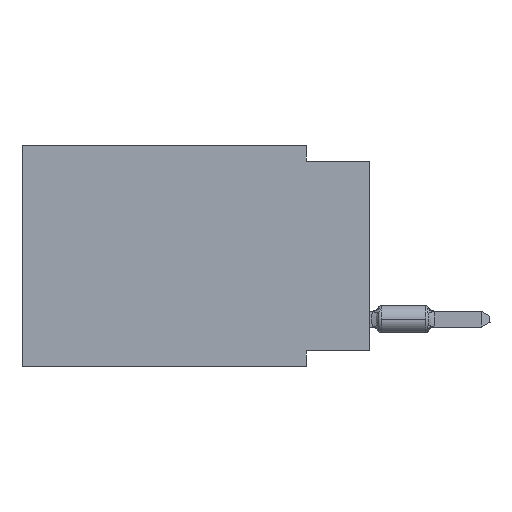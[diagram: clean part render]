
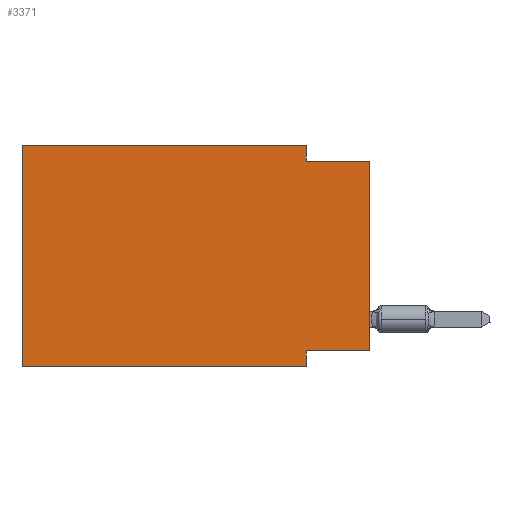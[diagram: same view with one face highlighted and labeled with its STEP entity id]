
A CAD part, left-side view. The second image highlights one B-rep face of the part: STEP entity #3371.
In plain terms, the highlighted planar face has unit normal (-1, 0, 0).
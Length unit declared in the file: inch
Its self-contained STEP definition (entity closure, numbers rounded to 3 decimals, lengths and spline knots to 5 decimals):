
#1636 = LINE ( 'NONE', #6308, #57875 ) ;
#3371 = ADVANCED_FACE ( 'NONE', ( #10774 ), #32274, .F. ) ;
#4884 = CARTESIAN_POINT ( 'NONE',  ( 0., 0., -0.325 ) ) ;
#5428 = DIRECTION ( 'NONE',  ( 0., 0., -1. ) ) ;
#6308 = CARTESIAN_POINT ( 'NONE',  ( 0., 0.55, -0.35 ) ) ;
#6967 = ORIENTED_EDGE ( 'NONE', *, *, #47789, .T. ) ;
#7202 = CARTESIAN_POINT ( 'NONE',  ( 0., 0.1, -0.35 ) ) ;
#7401 = CARTESIAN_POINT ( 'NONE',  ( 0., 0., -0.025 ) ) ;
#8218 = VECTOR ( 'NONE', #26713, 39.37008 ) ;
#8682 = DIRECTION ( 'NONE',  ( 0., -1., 0. ) ) ;
#9375 = DIRECTION ( 'NONE',  ( 0., 0., 1. ) ) ;
#9652 = VERTEX_POINT ( 'NONE', #34752 ) ;
#9842 = EDGE_CURVE ( 'NONE', #9652, #63638, #1636, .T. ) ;
#10419 = CARTESIAN_POINT ( 'NONE',  ( 0., 0., 0. ) ) ;
#10774 = FACE_OUTER_BOUND ( 'NONE', #28604, .T. ) ;
#10918 = EDGE_CURVE ( 'NONE', #28809, #63638, #18641, .T. ) ;
#11044 = EDGE_CURVE ( 'NONE', #39168, #31071, #43657, .T. ) ;
#12525 = LINE ( 'NONE', #45821, #33131 ) ;
#13208 = DIRECTION ( 'NONE',  ( 0., 0., 1. ) ) ;
#13335 = VECTOR ( 'NONE', #26827, 39.37008 ) ;
#14030 = LINE ( 'NONE', #35881, #62328 ) ;
#14391 = VERTEX_POINT ( 'NONE', #18608 ) ;
#14512 = VERTEX_POINT ( 'NONE', #43275 ) ;
#15196 = ORIENTED_EDGE ( 'NONE', *, *, #20431, .F. ) ;
#17984 = ORIENTED_EDGE ( 'NONE', *, *, #9842, .T. ) ;
#18608 = CARTESIAN_POINT ( 'NONE',  ( 0., 0.55, 0. ) ) ;
#18641 = LINE ( 'NONE', #7202, #36229 ) ;
#20431 = EDGE_CURVE ( 'NONE', #14391, #39168, #14030, .T. ) ;
#20669 = ORIENTED_EDGE ( 'NONE', *, *, #49768, .F. ) ;
#23967 = VERTEX_POINT ( 'NONE', #7401 ) ;
#24778 = VECTOR ( 'NONE', #13208, 39.37008 ) ;
#26538 = LINE ( 'NONE', #10419, #69568 ) ;
#26666 = CARTESIAN_POINT ( 'NONE',  ( 0., 0.1, 0. ) ) ;
#26713 = DIRECTION ( 'NONE',  ( 0., 1., 0. ) ) ;
#26827 = DIRECTION ( 'NONE',  ( 0., 0., -1. ) ) ;
#27787 = DIRECTION ( 'NONE',  ( 0., -1., 0. ) ) ;
#28604 = EDGE_LOOP ( 'NONE', ( #6967, #20669, #50465, #15196, #34947, #17984, #60137, #47807 ) ) ;
#28809 = VERTEX_POINT ( 'NONE', #62610 ) ;
#31071 = VERTEX_POINT ( 'NONE', #70292 ) ;
#32274 = PLANE ( 'NONE',  #36936 ) ;
#32628 = CARTESIAN_POINT ( 'NONE',  ( 0., 0.55, 0. ) ) ;
#33131 = VECTOR ( 'NONE', #40450, 39.37008 ) ;
#34414 = DIRECTION ( 'NONE',  ( 0., 0., -1. ) ) ;
#34752 = CARTESIAN_POINT ( 'NONE',  ( 0., 0.55, -0.35 ) ) ;
#34947 = ORIENTED_EDGE ( 'NONE', *, *, #70506, .F. ) ;
#35881 = CARTESIAN_POINT ( 'NONE',  ( 0., 0.55, 0. ) ) ;
#36229 = VECTOR ( 'NONE', #34414, 39.37008 ) ;
#36936 = AXIS2_PLACEMENT_3D ( 'NONE', #32628, #69927, #5428 ) ;
#39168 = VERTEX_POINT ( 'NONE', #26666 ) ;
#40450 = DIRECTION ( 'NONE',  ( 0., -1., 0. ) ) ;
#43275 = CARTESIAN_POINT ( 'NONE',  ( 0., 0., -0.325 ) ) ;
#43657 = LINE ( 'NONE', #44719, #13335 ) ;
#44147 = CARTESIAN_POINT ( 'NONE',  ( 0., 0.1, -0.35 ) ) ;
#44719 = CARTESIAN_POINT ( 'NONE',  ( 0., 0.1, 0. ) ) ;
#45821 = CARTESIAN_POINT ( 'NONE',  ( 0., 0., -0.025 ) ) ;
#47789 = EDGE_CURVE ( 'NONE', #14512, #23967, #26538, .T. ) ;
#47807 = ORIENTED_EDGE ( 'NONE', *, *, #59214, .F. ) ;
#49768 = EDGE_CURVE ( 'NONE', #31071, #23967, #12525, .T. ) ;
#50465 = ORIENTED_EDGE ( 'NONE', *, *, #11044, .F. ) ;
#53938 = LINE ( 'NONE', #4884, #8218 ) ;
#56917 = LINE ( 'NONE', #57990, #24778 ) ;
#57875 = VECTOR ( 'NONE', #27787, 39.37008 ) ;
#57990 = CARTESIAN_POINT ( 'NONE',  ( 0., 0.55, 0. ) ) ;
#59214 = EDGE_CURVE ( 'NONE', #14512, #28809, #53938, .T. ) ;
#60137 = ORIENTED_EDGE ( 'NONE', *, *, #10918, .F. ) ;
#62328 = VECTOR ( 'NONE', #8682, 39.37008 ) ;
#62610 = CARTESIAN_POINT ( 'NONE',  ( 0., 0.1, -0.325 ) ) ;
#63638 = VERTEX_POINT ( 'NONE', #44147 ) ;
#69568 = VECTOR ( 'NONE', #9375, 39.37008 ) ;
#69927 = DIRECTION ( 'NONE',  ( 1., 0., 0. ) ) ;
#70292 = CARTESIAN_POINT ( 'NONE',  ( 0., 0.1, -0.025 ) ) ;
#70506 = EDGE_CURVE ( 'NONE', #9652, #14391, #56917, .T. ) ;
